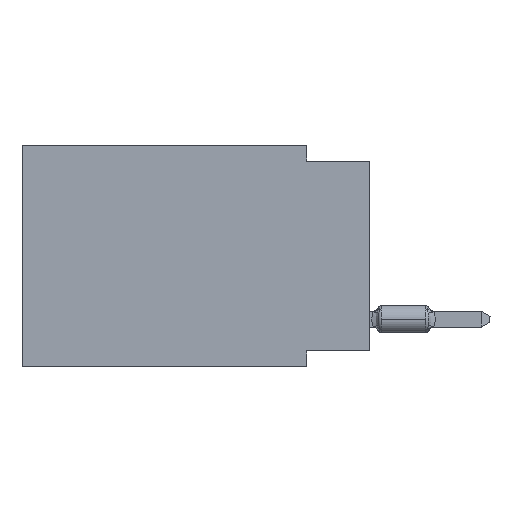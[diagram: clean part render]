
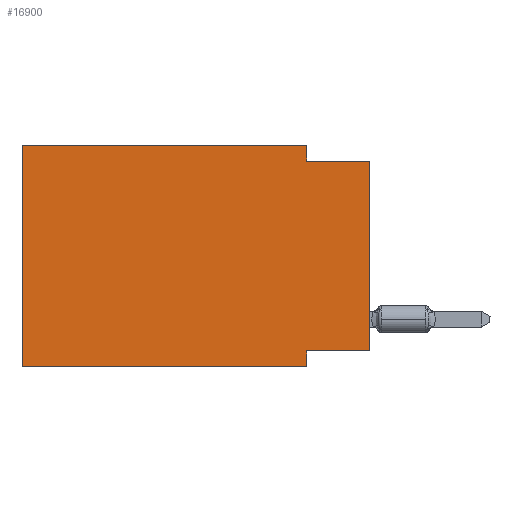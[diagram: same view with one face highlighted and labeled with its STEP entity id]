
A CAD part, left-side view. The second image highlights one B-rep face of the part: STEP entity #16900.
In plain terms, the highlighted planar face has unit normal (-1, 0, 0).
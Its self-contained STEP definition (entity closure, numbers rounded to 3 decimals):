
#358 = DIRECTION ( 'NONE',  ( 0., 0., -1. ) ) ;
#577 = CARTESIAN_POINT ( 'NONE',  ( 0., 0., -8.255 ) ) ;
#1631 = ORIENTED_EDGE ( 'NONE', *, *, #31432, .F. ) ;
#2882 = LINE ( 'NONE', #10233, #30743 ) ;
#3818 = DIRECTION ( 'NONE',  ( 0., 0., 1. ) ) ;
#4049 = ORIENTED_EDGE ( 'NONE', *, *, #12222, .F. ) ;
#4377 = VECTOR ( 'NONE', #3818, 1000. ) ;
#4764 = CARTESIAN_POINT ( 'NONE',  ( 0., 2.54, -8.89 ) ) ;
#4788 = EDGE_CURVE ( 'NONE', #27244, #22516, #19840, .T. ) ;
#5418 = AXIS2_PLACEMENT_3D ( 'NONE', #21184, #28677, #358 ) ;
#7970 = EDGE_CURVE ( 'NONE', #8361, #22516, #17433, .T. ) ;
#8361 = VERTEX_POINT ( 'NONE', #18057 ) ;
#8415 = LINE ( 'NONE', #577, #27019 ) ;
#9183 = ORIENTED_EDGE ( 'NONE', *, *, #30729, .T. ) ;
#9351 = EDGE_CURVE ( 'NONE', #17616, #25039, #30135, .T. ) ;
#9947 = CARTESIAN_POINT ( 'NONE',  ( 0., 13.97, 0. ) ) ;
#10233 = CARTESIAN_POINT ( 'NONE',  ( 0., 13.97, 0. ) ) ;
#10268 = VECTOR ( 'NONE', #25755, 1000. ) ;
#10288 = ORIENTED_EDGE ( 'NONE', *, *, #9351, .F. ) ;
#10761 = DIRECTION ( 'NONE',  ( 0., 1., 0. ) ) ;
#10790 = LINE ( 'NONE', #10950, #18025 ) ;
#10950 = CARTESIAN_POINT ( 'NONE',  ( 0., 2.54, 0. ) ) ;
#11024 = PLANE ( 'NONE',  #5418 ) ;
#11225 = ORIENTED_EDGE ( 'NONE', *, *, #22943, .F. ) ;
#12222 = EDGE_CURVE ( 'NONE', #29485, #8361, #8415, .T. ) ;
#12675 = ORIENTED_EDGE ( 'NONE', *, *, #4788, .T. ) ;
#13807 = EDGE_LOOP ( 'NONE', ( #9183, #10288, #31311, #1631, #11225, #12675, #20785, #4049 ) ) ;
#15722 = DIRECTION ( 'NONE',  ( 0., 0., 1. ) ) ;
#16650 = CARTESIAN_POINT ( 'NONE',  ( 0., 0., -8.255 ) ) ;
#16900 = ADVANCED_FACE ( 'NONE', ( #18689 ), #11024, .F. ) ;
#17105 = CARTESIAN_POINT ( 'NONE',  ( 0., 2.54, -8.89 ) ) ;
#17336 = DIRECTION ( 'NONE',  ( 0., -1., 0. ) ) ;
#17433 = LINE ( 'NONE', #4764, #29829 ) ;
#17616 = VERTEX_POINT ( 'NONE', #31409 ) ;
#18025 = VECTOR ( 'NONE', #21108, 1000. ) ;
#18057 = CARTESIAN_POINT ( 'NONE',  ( 0., 2.54, -8.255 ) ) ;
#18689 = FACE_OUTER_BOUND ( 'NONE', #13807, .T. ) ;
#18764 = VERTEX_POINT ( 'NONE', #22768 ) ;
#18825 = LINE ( 'NONE', #31659, #4377 ) ;
#19840 = LINE ( 'NONE', #32997, #23554 ) ;
#20141 = DIRECTION ( 'NONE',  ( 0., -1., 0. ) ) ;
#20785 = ORIENTED_EDGE ( 'NONE', *, *, #7970, .F. ) ;
#20981 = VERTEX_POINT ( 'NONE', #24335 ) ;
#21108 = DIRECTION ( 'NONE',  ( 0., 0., -1. ) ) ;
#21184 = CARTESIAN_POINT ( 'NONE',  ( 0., 13.97, 0. ) ) ;
#22516 = VERTEX_POINT ( 'NONE', #17105 ) ;
#22768 = CARTESIAN_POINT ( 'NONE',  ( 0., 2.54, 0. ) ) ;
#22943 = EDGE_CURVE ( 'NONE', #27244, #20981, #2882, .T. ) ;
#23415 = LINE ( 'NONE', #9947, #10268 ) ;
#23554 = VECTOR ( 'NONE', #17336, 1000. ) ;
#24335 = CARTESIAN_POINT ( 'NONE',  ( 0., 13.97, 0. ) ) ;
#24874 = EDGE_CURVE ( 'NONE', #18764, #17616, #10790, .T. ) ;
#25039 = VERTEX_POINT ( 'NONE', #27926 ) ;
#25755 = DIRECTION ( 'NONE',  ( 0., -1., 0. ) ) ;
#27019 = VECTOR ( 'NONE', #10761, 1000. ) ;
#27244 = VERTEX_POINT ( 'NONE', #29156 ) ;
#27591 = DIRECTION ( 'NONE',  ( 0., 0., -1. ) ) ;
#27926 = CARTESIAN_POINT ( 'NONE',  ( 0., 0., -0.635 ) ) ;
#27960 = CARTESIAN_POINT ( 'NONE',  ( 0., 0., -0.635 ) ) ;
#28677 = DIRECTION ( 'NONE',  ( 1., 0., 0. ) ) ;
#29156 = CARTESIAN_POINT ( 'NONE',  ( 0., 13.97, -8.89 ) ) ;
#29485 = VERTEX_POINT ( 'NONE', #16650 ) ;
#29829 = VECTOR ( 'NONE', #27591, 1000. ) ;
#30135 = LINE ( 'NONE', #27960, #31417 ) ;
#30729 = EDGE_CURVE ( 'NONE', #29485, #25039, #18825, .T. ) ;
#30743 = VECTOR ( 'NONE', #15722, 1000. ) ;
#31311 = ORIENTED_EDGE ( 'NONE', *, *, #24874, .F. ) ;
#31409 = CARTESIAN_POINT ( 'NONE',  ( 0., 2.54, -0.635 ) ) ;
#31417 = VECTOR ( 'NONE', #20141, 1000. ) ;
#31432 = EDGE_CURVE ( 'NONE', #20981, #18764, #23415, .T. ) ;
#31659 = CARTESIAN_POINT ( 'NONE',  ( 0., 0., 0. ) ) ;
#32997 = CARTESIAN_POINT ( 'NONE',  ( 0., 13.97, -8.89 ) ) ;
